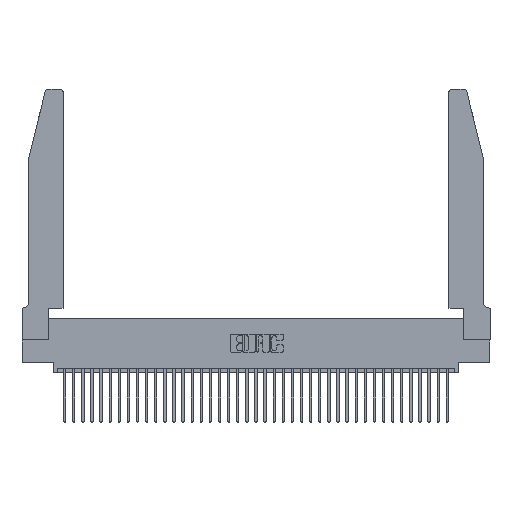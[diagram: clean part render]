
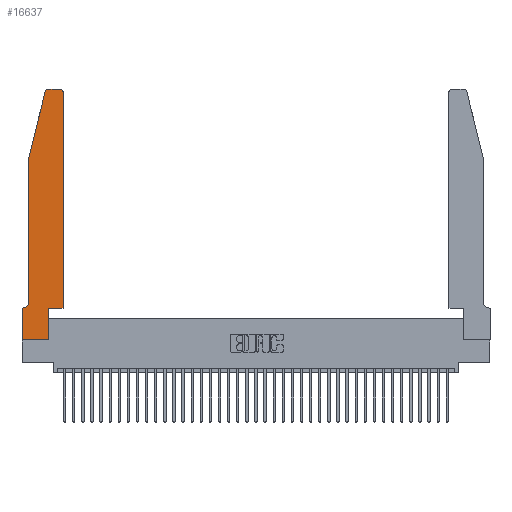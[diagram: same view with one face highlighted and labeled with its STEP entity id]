
A CAD part, top view. The second image highlights one B-rep face of the part: STEP entity #16637.
In plain terms, the highlighted planar face has unit normal (0, 0, 1).
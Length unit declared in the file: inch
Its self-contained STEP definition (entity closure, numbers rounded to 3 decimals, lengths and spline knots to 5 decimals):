
#1290 = LINE ( 'NONE', #17594, #9255 ) ;
#1873 = DIRECTION ( 'NONE',  ( -1., 0., 0. ) ) ;
#2006 = CARTESIAN_POINT ( 'NONE',  ( 0.4505, 0.35, 0.37 ) ) ;
#2172 = CARTESIAN_POINT ( 'NONE',  ( 0.0755, 2., 0.37 ) ) ;
#2260 = CARTESIAN_POINT ( 'NONE',  ( 0., 0., 0.37 ) ) ;
#2482 = LINE ( 'NONE', #17913, #35491 ) ;
#2903 = VERTEX_POINT ( 'NONE', #14264 ) ;
#2963 = DIRECTION ( 'NONE',  ( 1., 0., 0. ) ) ;
#3027 = DIRECTION ( 'NONE',  ( 0., 0., 1. ) ) ;
#3045 = EDGE_CURVE ( 'NONE', #24879, #16688, #18298, .T. ) ;
#3501 = AXIS2_PLACEMENT_3D ( 'NONE', #16488, #3027, #7813 ) ;
#4162 = ORIENTED_EDGE ( 'NONE', *, *, #17474, .T. ) ;
#4790 = AXIS2_PLACEMENT_3D ( 'NONE', #25224, #31175, #34189 ) ;
#4927 = ORIENTED_EDGE ( 'NONE', *, *, #30149, .T. ) ;
#5261 = CARTESIAN_POINT ( 'NONE',  ( 0.0755, 2., 0.37 ) ) ;
#5745 = VERTEX_POINT ( 'NONE', #16323 ) ;
#6300 = ORIENTED_EDGE ( 'NONE', *, *, #7503, .T. ) ;
#6488 = EDGE_CURVE ( 'NONE', #16688, #20119, #1290, .T. ) ;
#6899 = CARTESIAN_POINT ( 'NONE',  ( 0.284, 2.75, 0.37 ) ) ;
#7136 = AXIS2_PLACEMENT_3D ( 'NONE', #28140, #10320, #36670 ) ;
#7503 = EDGE_CURVE ( 'NONE', #20119, #34378, #12876, .T. ) ;
#7813 = DIRECTION ( 'NONE',  ( 1., 0., 0. ) ) ;
#7970 = CIRCLE ( 'NONE', #3501, 0.03 ) ;
#8285 = VECTOR ( 'NONE', #10824, 39.37008 ) ;
#8425 = DIRECTION ( 'NONE',  ( -0.239, -0.971, 0. ) ) ;
#9255 = VECTOR ( 'NONE', #17850, 39.37008 ) ;
#9296 = AXIS2_PLACEMENT_3D ( 'NONE', #17027, #20771, #2963 ) ;
#10320 = DIRECTION ( 'NONE',  ( 0., 0., -1. ) ) ;
#10508 = VERTEX_POINT ( 'NONE', #2172 ) ;
#10824 = DIRECTION ( 'NONE',  ( 0., -1., 0. ) ) ;
#11220 = CARTESIAN_POINT ( 'NONE',  ( 0., 0., 0.37 ) ) ;
#11422 = ORIENTED_EDGE ( 'NONE', *, *, #24918, .T. ) ;
#11509 = CIRCLE ( 'NONE', #7136, 0.07 ) ;
#12530 = EDGE_CURVE ( 'NONE', #29191, #24879, #11509, .T. ) ;
#12782 = ORIENTED_EDGE ( 'NONE', *, *, #15320, .T. ) ;
#12876 = LINE ( 'NONE', #11220, #27760 ) ;
#13200 = CARTESIAN_POINT ( 'NONE',  ( 0.25487, 2.72718, 0.37 ) ) ;
#13204 = LINE ( 'NONE', #24930, #21526 ) ;
#13418 = VECTOR ( 'NONE', #20528, 39.37008 ) ;
#13942 = DIRECTION ( 'NONE',  ( -1., 0., 0. ) ) ;
#14264 = CARTESIAN_POINT ( 'NONE',  ( 0.4205, 2.75, 0.37 ) ) ;
#14997 = DIRECTION ( 'NONE',  ( 1., 0., 0. ) ) ;
#15320 = EDGE_CURVE ( 'NONE', #35648, #24430, #36482, .T. ) ;
#16323 = CARTESIAN_POINT ( 'NONE',  ( 0.2865, 0.35, 0.37 ) ) ;
#16488 = CARTESIAN_POINT ( 'NONE',  ( 0.4205, 2.72, 0.37 ) ) ;
#16551 = DIRECTION ( 'NONE',  ( 0., 1., 0. ) ) ;
#16637 = ADVANCED_FACE ( 'NONE', ( #26255 ), #31896, .T. ) ;
#16688 = VERTEX_POINT ( 'NONE', #37752 ) ;
#17027 = CARTESIAN_POINT ( 'NONE',  ( 0., 0.35, 0.37 ) ) ;
#17174 = CARTESIAN_POINT ( 'NONE',  ( 0.4505, 0.35, 0.37 ) ) ;
#17474 = EDGE_CURVE ( 'NONE', #5745, #35648, #13204, .T. ) ;
#17594 = CARTESIAN_POINT ( 'NONE',  ( 0., 0., 0.37 ) ) ;
#17850 = DIRECTION ( 'NONE',  ( 0., -1., 0. ) ) ;
#17913 = CARTESIAN_POINT ( 'NONE',  ( 0.0755, 2., 0.37 ) ) ;
#17946 = VECTOR ( 'NONE', #16551, 39.37008 ) ;
#18298 = LINE ( 'NONE', #24741, #32197 ) ;
#19512 = CARTESIAN_POINT ( 'NONE',  ( 0.4505, 2.72, 0.37 ) ) ;
#19527 = CIRCLE ( 'NONE', #4790, 0.03 ) ;
#20119 = VERTEX_POINT ( 'NONE', #2260 ) ;
#20236 = ORIENTED_EDGE ( 'NONE', *, *, #27087, .T. ) ;
#20329 = VECTOR ( 'NONE', #1873, 39.37008 ) ;
#20528 = DIRECTION ( 'NONE',  ( 0., 1., 0. ) ) ;
#20771 = DIRECTION ( 'NONE',  ( 0., 0., 1. ) ) ;
#20828 = LINE ( 'NONE', #5261, #8285 ) ;
#20943 = ORIENTED_EDGE ( 'NONE', *, *, #12530, .T. ) ;
#21526 = VECTOR ( 'NONE', #29951, 39.37008 ) ;
#23844 = ORIENTED_EDGE ( 'NONE', *, *, #3045, .T. ) ;
#23932 = CARTESIAN_POINT ( 'NONE',  ( 0.0755, 0.42, 0.37 ) ) ;
#24430 = VERTEX_POINT ( 'NONE', #19512 ) ;
#24741 = CARTESIAN_POINT ( 'NONE',  ( 0.0755, 0.35, 0.37 ) ) ;
#24879 = VERTEX_POINT ( 'NONE', #26491 ) ;
#24918 = EDGE_CURVE ( 'NONE', #25048, #10508, #2482, .T. ) ;
#24930 = CARTESIAN_POINT ( 'NONE',  ( 0.4505, 0.35, 0.37 ) ) ;
#25048 = VERTEX_POINT ( 'NONE', #13200 ) ;
#25224 = CARTESIAN_POINT ( 'NONE',  ( 0.284, 2.72, 0.37 ) ) ;
#25569 = CARTESIAN_POINT ( 'NONE',  ( 0.2605, 2.75, 0.37 ) ) ;
#26255 = FACE_OUTER_BOUND ( 'NONE', #34241, .T. ) ;
#26465 = LINE ( 'NONE', #32594, #13418 ) ;
#26491 = CARTESIAN_POINT ( 'NONE',  ( 0.0055, 0.35, 0.37 ) ) ;
#27087 = EDGE_CURVE ( 'NONE', #24430, #2903, #7970, .T. ) ;
#27352 = ORIENTED_EDGE ( 'NONE', *, *, #29657, .T. ) ;
#27760 = VECTOR ( 'NONE', #14997, 39.37008 ) ;
#28140 = CARTESIAN_POINT ( 'NONE',  ( 0.0055, 0.42, 0.37 ) ) ;
#28641 = EDGE_CURVE ( 'NONE', #32646, #25048, #19527, .T. ) ;
#29191 = VERTEX_POINT ( 'NONE', #23932 ) ;
#29657 = EDGE_CURVE ( 'NONE', #34378, #5745, #26465, .T. ) ;
#29951 = DIRECTION ( 'NONE',  ( 1., 0., 0. ) ) ;
#30149 = EDGE_CURVE ( 'NONE', #10508, #29191, #20828, .T. ) ;
#31175 = DIRECTION ( 'NONE',  ( 0., 0., 1. ) ) ;
#31896 = PLANE ( 'NONE',  #9296 ) ;
#32197 = VECTOR ( 'NONE', #13942, 39.37008 ) ;
#32528 = ORIENTED_EDGE ( 'NONE', *, *, #35607, .T. ) ;
#32594 = CARTESIAN_POINT ( 'NONE',  ( 0.2865, 0.35, 0.37 ) ) ;
#32646 = VERTEX_POINT ( 'NONE', #6899 ) ;
#33326 = LINE ( 'NONE', #25569, #20329 ) ;
#34189 = DIRECTION ( 'NONE',  ( 1., 0., 0. ) ) ;
#34241 = EDGE_LOOP ( 'NONE', ( #32528, #35789, #11422, #4927, #20943, #23844, #36463, #6300, #27352, #4162, #12782, #20236 ) ) ;
#34378 = VERTEX_POINT ( 'NONE', #38243 ) ;
#35491 = VECTOR ( 'NONE', #8425, 39.37008 ) ;
#35607 = EDGE_CURVE ( 'NONE', #2903, #32646, #33326, .T. ) ;
#35648 = VERTEX_POINT ( 'NONE', #2006 ) ;
#35789 = ORIENTED_EDGE ( 'NONE', *, *, #28641, .T. ) ;
#36463 = ORIENTED_EDGE ( 'NONE', *, *, #6488, .T. ) ;
#36482 = LINE ( 'NONE', #17174, #17946 ) ;
#36670 = DIRECTION ( 'NONE',  ( -1., 0., 0. ) ) ;
#37752 = CARTESIAN_POINT ( 'NONE',  ( 0., 0.35, 0.37 ) ) ;
#38243 = CARTESIAN_POINT ( 'NONE',  ( 0.2865, 0., 0.37 ) ) ;
